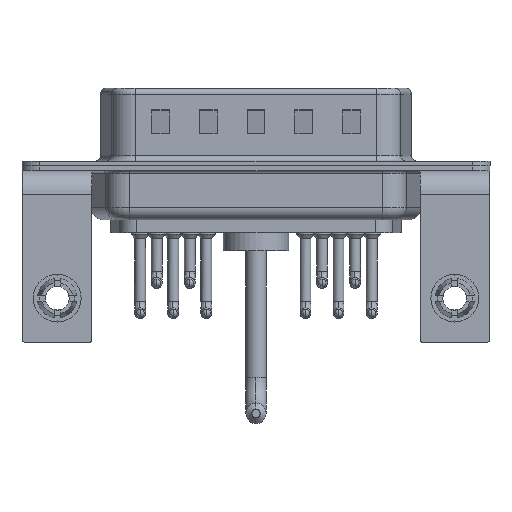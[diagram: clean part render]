
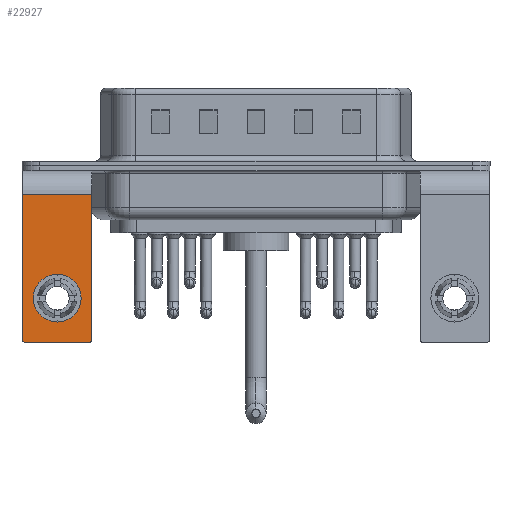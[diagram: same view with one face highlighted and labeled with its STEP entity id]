
A CAD part, front view. The second image highlights one B-rep face of the part: STEP entity #22927.
In plain terms, the highlighted planar face has unit normal (0, -1, 0).
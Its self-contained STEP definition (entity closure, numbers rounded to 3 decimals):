
#1445 = VERTEX_POINT ( 'NONE', #8721 ) ;
#1550 = CARTESIAN_POINT ( 'NONE',  ( 2.9, -6.25, -14.55 ) ) ;
#1797 = DIRECTION ( 'NONE',  ( 0., 0., -1. ) ) ;
#1955 = DIRECTION ( 'NONE',  ( 0., 0., 1. ) ) ;
#2326 = CARTESIAN_POINT ( 'NONE',  ( 0., -6.25, -11.07 ) ) ;
#2416 = CARTESIAN_POINT ( 'NONE',  ( -2.65, -6.25, -14.8 ) ) ;
#2562 = EDGE_CURVE ( 'NONE', #18751, #22147, #23997, .T. ) ;
#3096 = EDGE_CURVE ( 'NONE', #8060, #7347, #15988, .T. ) ;
#4540 = AXIS2_PLACEMENT_3D ( 'NONE', #2326, #23256, #9882 ) ;
#4774 = CARTESIAN_POINT ( 'NONE',  ( 2.9, -6.25, -2.4 ) ) ;
#4775 = EDGE_CURVE ( 'NONE', #1445, #8060, #24710, .T. ) ;
#6106 = CARTESIAN_POINT ( 'NONE',  ( -2.65, -6.25, -14.55 ) ) ;
#6452 = VECTOR ( 'NONE', #17263, 1000. ) ;
#6657 = FACE_BOUND ( 'NONE', #12516, .T. ) ;
#6916 = FACE_OUTER_BOUND ( 'NONE', #23335, .T. ) ;
#7150 = CARTESIAN_POINT ( 'NONE',  ( 2.65, -6.25, -14.8 ) ) ;
#7176 = ORIENTED_EDGE ( 'NONE', *, *, #19696, .F. ) ;
#7347 = VERTEX_POINT ( 'NONE', #18608 ) ;
#7709 = EDGE_CURVE ( 'NONE', #1445, #22147, #12761, .T. ) ;
#7869 = AXIS2_PLACEMENT_3D ( 'NONE', #21956, #19220, #1955 ) ;
#8030 = ORIENTED_EDGE ( 'NONE', *, *, #3096, .T. ) ;
#8060 = VERTEX_POINT ( 'NONE', #10219 ) ;
#8414 = ORIENTED_EDGE ( 'NONE', *, *, #11857, .T. ) ;
#8721 = CARTESIAN_POINT ( 'NONE',  ( 2.9, -6.25, -2.4 ) ) ;
#9743 = ORIENTED_EDGE ( 'NONE', *, *, #7709, .F. ) ;
#9882 = DIRECTION ( 'NONE',  ( 0., 0., 1. ) ) ;
#9947 = CARTESIAN_POINT ( 'NONE',  ( -2.9, -6.25, -2.4 ) ) ;
#10102 = DIRECTION ( 'NONE',  ( 0., 1., 0. ) ) ;
#10219 = CARTESIAN_POINT ( 'NONE',  ( -2.9, -6.25, -2.4 ) ) ;
#10538 = VERTEX_POINT ( 'NONE', #2416 ) ;
#10559 = DIRECTION ( 'NONE',  ( 0., 1., 0. ) ) ;
#11313 = CIRCLE ( 'NONE', #19378, 0.25 ) ;
#11695 = CARTESIAN_POINT ( 'NONE',  ( 0., -6.25, -9.07 ) ) ;
#11702 = CARTESIAN_POINT ( 'NONE',  ( 2.9, -6.25, -14.8 ) ) ;
#11739 = CARTESIAN_POINT ( 'NONE',  ( 0., -6.25, -11.07 ) ) ;
#11857 = EDGE_CURVE ( 'NONE', #7347, #10538, #11313, .T. ) ;
#12053 = ORIENTED_EDGE ( 'NONE', *, *, #4775, .T. ) ;
#12177 = AXIS2_PLACEMENT_3D ( 'NONE', #11739, #10102, #13514 ) ;
#12254 = ORIENTED_EDGE ( 'NONE', *, *, #13159, .T. ) ;
#12516 = EDGE_LOOP ( 'NONE', ( #12254, #15779 ) ) ;
#12761 = LINE ( 'NONE', #24633, #22075 ) ;
#13159 = EDGE_CURVE ( 'NONE', #15436, #18467, #21456, .T. ) ;
#13381 = VECTOR ( 'NONE', #23693, 1000. ) ;
#13514 = DIRECTION ( 'NONE',  ( 0., 0., 1. ) ) ;
#13574 = EDGE_CURVE ( 'NONE', #18467, #15436, #23079, .T. ) ;
#13662 = DIRECTION ( 'NONE',  ( 0., -1., 0. ) ) ;
#14344 = DIRECTION ( 'NONE',  ( 0., 0., 1. ) ) ;
#14843 = PLANE ( 'NONE',  #23034 ) ;
#15436 = VERTEX_POINT ( 'NONE', #20767 ) ;
#15779 = ORIENTED_EDGE ( 'NONE', *, *, #13574, .T. ) ;
#15988 = LINE ( 'NONE', #9947, #13381 ) ;
#17263 = DIRECTION ( 'NONE',  ( -1., 0., 0. ) ) ;
#18467 = VERTEX_POINT ( 'NONE', #11695 ) ;
#18608 = CARTESIAN_POINT ( 'NONE',  ( -2.9, -6.25, -14.55 ) ) ;
#18751 = VERTEX_POINT ( 'NONE', #7150 ) ;
#18830 = ORIENTED_EDGE ( 'NONE', *, *, #2562, .T. ) ;
#18897 = CARTESIAN_POINT ( 'NONE',  ( 2.9, -6.25, -2.4 ) ) ;
#19145 = DIRECTION ( 'NONE',  ( -1., 0., 0. ) ) ;
#19220 = DIRECTION ( 'NONE',  ( 0., -1., 0. ) ) ;
#19378 = AXIS2_PLACEMENT_3D ( 'NONE', #6106, #13662, #23622 ) ;
#19696 = EDGE_CURVE ( 'NONE', #18751, #10538, #22815, .T. ) ;
#20767 = CARTESIAN_POINT ( 'NONE',  ( 0., -6.25, -13.07 ) ) ;
#21456 = CIRCLE ( 'NONE', #4540, 2. ) ;
#21956 = CARTESIAN_POINT ( 'NONE',  ( 2.65, -6.25, -14.55 ) ) ;
#22075 = VECTOR ( 'NONE', #1797, 1000. ) ;
#22147 = VERTEX_POINT ( 'NONE', #1550 ) ;
#22815 = LINE ( 'NONE', #11702, #6452 ) ;
#22927 = ADVANCED_FACE ( 'NONE', ( #6657, #6916 ), #14843, .F. ) ;
#23034 = AXIS2_PLACEMENT_3D ( 'NONE', #4774, #10559, #14344 ) ;
#23079 = CIRCLE ( 'NONE', #12177, 2. ) ;
#23256 = DIRECTION ( 'NONE',  ( 0., 1., 0. ) ) ;
#23335 = EDGE_LOOP ( 'NONE', ( #8030, #8414, #7176, #18830, #9743, #12053 ) ) ;
#23622 = DIRECTION ( 'NONE',  ( 0., 0., 1. ) ) ;
#23693 = DIRECTION ( 'NONE',  ( 0., 0., -1. ) ) ;
#23997 = CIRCLE ( 'NONE', #7869, 0.25 ) ;
#24633 = CARTESIAN_POINT ( 'NONE',  ( 2.9, -6.25, -2.4 ) ) ;
#24710 = LINE ( 'NONE', #18897, #24857 ) ;
#24857 = VECTOR ( 'NONE', #19145, 1000. ) ;
